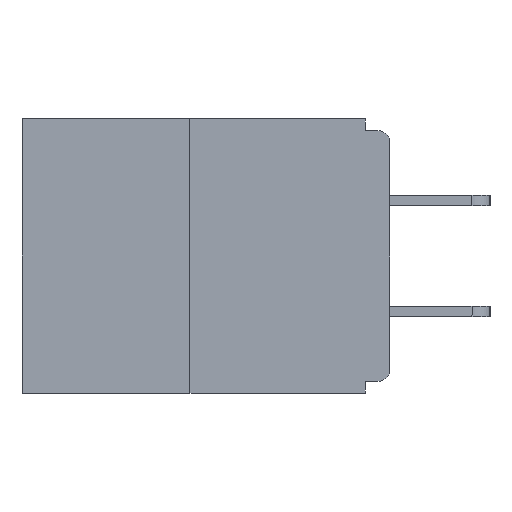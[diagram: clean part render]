
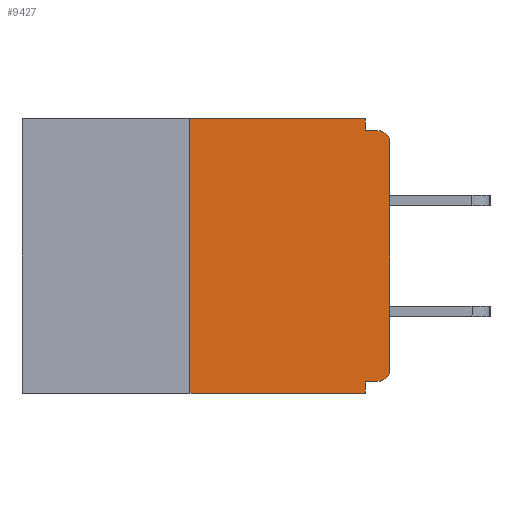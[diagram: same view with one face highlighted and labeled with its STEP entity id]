
A CAD part, left-side view. The second image highlights one B-rep face of the part: STEP entity #9427.
In plain terms, the highlighted planar face has unit normal (-1, 0, 0).
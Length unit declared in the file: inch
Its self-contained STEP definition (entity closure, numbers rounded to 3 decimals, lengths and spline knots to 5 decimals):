
#12 = VERTEX_POINT ( 'NONE', #5409 ) ;
#69 = AXIS2_PLACEMENT_3D ( 'NONE', #11010, #8405, #3232 ) ;
#156 = VECTOR ( 'NONE', #5176, 39.37008 ) ;
#549 = DIRECTION ( 'NONE',  ( 0., 0., 1. ) ) ;
#748 = VECTOR ( 'NONE', #5336, 39.37008 ) ;
#962 = VERTEX_POINT ( 'NONE', #10589 ) ;
#1007 = LINE ( 'NONE', #5614, #8044 ) ;
#1335 = LINE ( 'NONE', #10934, #10255 ) ;
#1409 = PLANE ( 'NONE',  #3631 ) ;
#1558 = DIRECTION ( 'NONE',  ( 0., 0., -1. ) ) ;
#1595 = CARTESIAN_POINT ( 'NONE',  ( 0., 0.031, 0. ) ) ;
#1709 = DIRECTION ( 'NONE',  ( -1., 0., 0. ) ) ;
#1749 = CARTESIAN_POINT ( 'NONE',  ( 0., 0.25, -0.343 ) ) ;
#1846 = ORIENTED_EDGE ( 'NONE', *, *, #10475, .T. ) ;
#1865 = VECTOR ( 'NONE', #4356, 39.37008 ) ;
#1900 = VERTEX_POINT ( 'NONE', #3194 ) ;
#1912 = VERTEX_POINT ( 'NONE', #7550 ) ;
#1998 = CIRCLE ( 'NONE', #69, 0.015 ) ;
#2009 = EDGE_CURVE ( 'NONE', #962, #8086, #6743, .T. ) ;
#2140 = DIRECTION ( 'NONE',  ( 0., -1., 0. ) ) ;
#2292 = CARTESIAN_POINT ( 'NONE',  ( 0., 0.031, -0.015 ) ) ;
#2325 = ORIENTED_EDGE ( 'NONE', *, *, #9460, .F. ) ;
#2386 = VECTOR ( 'NONE', #7203, 39.37008 ) ;
#2406 = DIRECTION ( 'NONE',  ( 0., 0., -1. ) ) ;
#2784 = EDGE_CURVE ( 'NONE', #3253, #12, #1007, .T. ) ;
#2957 = CARTESIAN_POINT ( 'NONE',  ( 0., 0., -0.313 ) ) ;
#3037 = ORIENTED_EDGE ( 'NONE', *, *, #10977, .F. ) ;
#3089 = EDGE_CURVE ( 'NONE', #1900, #5133, #3864, .T. ) ;
#3140 = EDGE_CURVE ( 'NONE', #3951, #4533, #10057, .T. ) ;
#3194 = CARTESIAN_POINT ( 'NONE',  ( 0., 0.25, 0. ) ) ;
#3232 = DIRECTION ( 'NONE',  ( 0., 0., -1. ) ) ;
#3253 = VERTEX_POINT ( 'NONE', #2292 ) ;
#3350 = CARTESIAN_POINT ( 'NONE',  ( 0., 0.031, -0.343 ) ) ;
#3631 = AXIS2_PLACEMENT_3D ( 'NONE', #4133, #6835, #2406 ) ;
#3864 = LINE ( 'NONE', #4521, #5625 ) ;
#3951 = VERTEX_POINT ( 'NONE', #1749 ) ;
#4133 = CARTESIAN_POINT ( 'NONE',  ( 0., 0.46, 0. ) ) ;
#4356 = DIRECTION ( 'NONE',  ( 0., 1., 0. ) ) ;
#4521 = CARTESIAN_POINT ( 'NONE',  ( 0., 0.46, 0. ) ) ;
#4533 = VERTEX_POINT ( 'NONE', #9331 ) ;
#4945 = ORIENTED_EDGE ( 'NONE', *, *, #3140, .T. ) ;
#5133 = VERTEX_POINT ( 'NONE', #9816 ) ;
#5176 = DIRECTION ( 'NONE',  ( 0., 0., -1. ) ) ;
#5336 = DIRECTION ( 'NONE',  ( 0., 0., 1. ) ) ;
#5409 = CARTESIAN_POINT ( 'NONE',  ( 0., 0.015, -0.015 ) ) ;
#5506 = LINE ( 'NONE', #9672, #748 ) ;
#5614 = CARTESIAN_POINT ( 'NONE',  ( 0., 0., -0.015 ) ) ;
#5625 = VECTOR ( 'NONE', #10564, 39.37008 ) ;
#6057 = ORIENTED_EDGE ( 'NONE', *, *, #7971, .T. ) ;
#6260 = EDGE_CURVE ( 'NONE', #11091, #1912, #1335, .T. ) ;
#6289 = CARTESIAN_POINT ( 'NONE',  ( 0., 0.46, -0.343 ) ) ;
#6433 = FACE_OUTER_BOUND ( 'NONE', #6990, .T. ) ;
#6743 = LINE ( 'NONE', #9512, #1865 ) ;
#6817 = CARTESIAN_POINT ( 'NONE',  ( 0., 0.031, -0.328 ) ) ;
#6835 = DIRECTION ( 'NONE',  ( 1., 0., 0. ) ) ;
#6990 = EDGE_LOOP ( 'NONE', ( #7577, #7267, #4945, #3037, #9075, #1846, #7530, #6057, #8657, #2325 ) ) ;
#7203 = DIRECTION ( 'NONE',  ( 0., -1., 0. ) ) ;
#7267 = ORIENTED_EDGE ( 'NONE', *, *, #8331, .F. ) ;
#7530 = ORIENTED_EDGE ( 'NONE', *, *, #6260, .T. ) ;
#7550 = CARTESIAN_POINT ( 'NONE',  ( 0., 0., -0.03 ) ) ;
#7577 = ORIENTED_EDGE ( 'NONE', *, *, #3089, .F. ) ;
#7644 = DIRECTION ( 'NONE',  ( 0., 0., -1. ) ) ;
#7971 = EDGE_CURVE ( 'NONE', #1912, #12, #1998, .T. ) ;
#8044 = VECTOR ( 'NONE', #2140, 39.37008 ) ;
#8086 = VERTEX_POINT ( 'NONE', #6817 ) ;
#8331 = EDGE_CURVE ( 'NONE', #3951, #1900, #5506, .T. ) ;
#8405 = DIRECTION ( 'NONE',  ( -1., 0., 0. ) ) ;
#8657 = ORIENTED_EDGE ( 'NONE', *, *, #2784, .F. ) ;
#8800 = CIRCLE ( 'NONE', #10289, 0.015 ) ;
#9075 = ORIENTED_EDGE ( 'NONE', *, *, #2009, .F. ) ;
#9331 = CARTESIAN_POINT ( 'NONE',  ( 0., 0.031, -0.343 ) ) ;
#9427 = ADVANCED_FACE ( 'NONE', ( #6433 ), #1409, .F. ) ;
#9460 = EDGE_CURVE ( 'NONE', #5133, #3253, #11133, .T. ) ;
#9512 = CARTESIAN_POINT ( 'NONE',  ( 0., 0., -0.328 ) ) ;
#9672 = CARTESIAN_POINT ( 'NONE',  ( 0., 0.25, 0. ) ) ;
#9816 = CARTESIAN_POINT ( 'NONE',  ( 0., 0.031, 0. ) ) ;
#10057 = LINE ( 'NONE', #6289, #2386 ) ;
#10255 = VECTOR ( 'NONE', #549, 39.37008 ) ;
#10289 = AXIS2_PLACEMENT_3D ( 'NONE', #11142, #1709, #7644 ) ;
#10475 = EDGE_CURVE ( 'NONE', #962, #11091, #8800, .T. ) ;
#10564 = DIRECTION ( 'NONE',  ( 0., -1., 0. ) ) ;
#10589 = CARTESIAN_POINT ( 'NONE',  ( 0., 0.015, -0.328 ) ) ;
#10873 = VECTOR ( 'NONE', #1558, 39.37008 ) ;
#10934 = CARTESIAN_POINT ( 'NONE',  ( 0., 0., 0. ) ) ;
#10957 = LINE ( 'NONE', #3350, #156 ) ;
#10977 = EDGE_CURVE ( 'NONE', #8086, #4533, #10957, .T. ) ;
#11010 = CARTESIAN_POINT ( 'NONE',  ( 0., 0.015, -0.03 ) ) ;
#11091 = VERTEX_POINT ( 'NONE', #2957 ) ;
#11133 = LINE ( 'NONE', #1595, #10873 ) ;
#11142 = CARTESIAN_POINT ( 'NONE',  ( 0., 0.015, -0.313 ) ) ;
